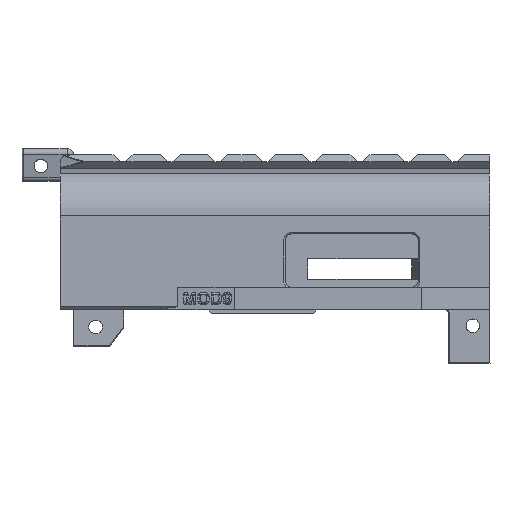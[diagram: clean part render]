
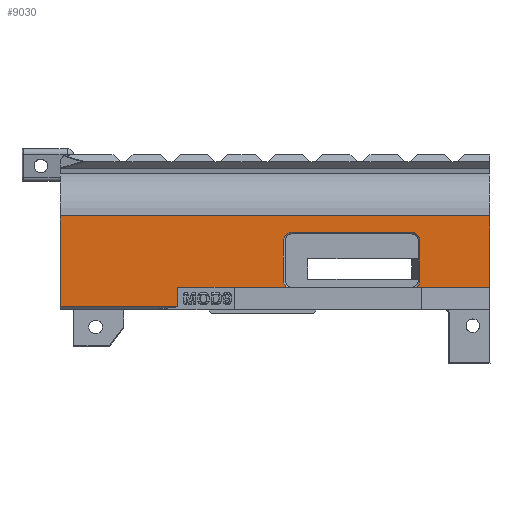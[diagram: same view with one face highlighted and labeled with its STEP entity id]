
A CAD part, top view. The second image highlights one B-rep face of the part: STEP entity #9030.
In plain terms, the highlighted planar face has unit normal (0, 0, 1).
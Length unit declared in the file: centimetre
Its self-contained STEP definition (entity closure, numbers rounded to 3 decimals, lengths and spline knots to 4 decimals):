
#732=LINE($,#12046,#1585);
#785=LINE($,#13323,#1638);
#786=LINE($,#13325,#1639);
#787=LINE($,#13328,#1640);
#788=LINE($,#13330,#1641);
#789=LINE($,#13332,#1642);
#790=LINE($,#13334,#1643);
#791=LINE($,#13336,#1644);
#792=LINE($,#13338,#1645);
#793=LINE($,#13342,#1646);
#794=LINE($,#13346,#1647);
#1585=VECTOR($,#10150,3.155);
#1638=VECTOR($,#10241,0.7183);
#1639=VECTOR($,#10242,1.0403);
#1640=VECTOR($,#10245,3.2523);
#1641=VECTOR($,#10246,19.0382);
#1642=VECTOR($,#10247,4.0257);
#1643=VECTOR($,#10248,5.189);
#1644=VECTOR($,#10249,0.8707);
#1645=VECTOR($,#10250,4.846);
#1646=VECTOR($,#10253,1.7606);
#1647=VECTOR($,#10256,5.2844);
#2394=PLANE($,#9542);
#2758=FACE_OUTER_BOUND($,#3283,.T.);
#3283=EDGE_LOOP($,(#6561,#6562,#6563,#6564,#6565,#6566,#6567,#6568,#6569,
#6570,#6571,#6572,#6573,#6574,#6575));
#3797=CIRCLE($,#9543,0.38);
#3798=CIRCLE($,#9544,0.38);
#3799=CIRCLE($,#9545,0.38);
#3800=CIRCLE($,#9546,0.38);
#3970=VERTEX_POINT($,#12043);
#3971=VERTEX_POINT($,#12045);
#4075=VERTEX_POINT($,#13321);
#4076=VERTEX_POINT($,#13322);
#4077=VERTEX_POINT($,#13324);
#4078=VERTEX_POINT($,#13326);
#4079=VERTEX_POINT($,#13329);
#4080=VERTEX_POINT($,#13331);
#4081=VERTEX_POINT($,#13333);
#4082=VERTEX_POINT($,#13335);
#4083=VERTEX_POINT($,#13337);
#4084=VERTEX_POINT($,#13339);
#4085=VERTEX_POINT($,#13341);
#4086=VERTEX_POINT($,#13343);
#4087=VERTEX_POINT($,#13345);
#4896=EDGE_CURVE($,#3971,#3970,#732,.T.);
#5046=EDGE_CURVE($,#4075,#4076,#785,.T.);
#5047=EDGE_CURVE($,#4077,#4075,#786,.T.);
#5048=EDGE_CURVE($,#4078,#4077,#3797,.T.);
#5049=EDGE_CURVE($,#3971,#4078,#787,.T.);
#5050=EDGE_CURVE($,#3970,#4079,#788,.T.);
#5051=EDGE_CURVE($,#4079,#4080,#789,.T.);
#5052=EDGE_CURVE($,#4081,#4080,#790,.T.);
#5053=EDGE_CURVE($,#4081,#4082,#791,.T.);
#5054=EDGE_CURVE($,#4083,#4082,#792,.T.);
#5055=EDGE_CURVE($,#4084,#4083,#3798,.T.);
#5056=EDGE_CURVE($,#4084,#4085,#793,.T.);
#5057=EDGE_CURVE($,#4086,#4085,#3799,.T.);
#5058=EDGE_CURVE($,#4087,#4086,#794,.T.);
#5059=EDGE_CURVE($,#4076,#4087,#3800,.T.);
#6561=ORIENTED_EDGE($,*,*,#5046,.F.);
#6562=ORIENTED_EDGE($,*,*,#5047,.F.);
#6563=ORIENTED_EDGE($,*,*,#5048,.F.);
#6564=ORIENTED_EDGE($,*,*,#5049,.F.);
#6565=ORIENTED_EDGE($,*,*,#4896,.T.);
#6566=ORIENTED_EDGE($,*,*,#5050,.T.);
#6567=ORIENTED_EDGE($,*,*,#5051,.T.);
#6568=ORIENTED_EDGE($,*,*,#5052,.F.);
#6569=ORIENTED_EDGE($,*,*,#5053,.T.);
#6570=ORIENTED_EDGE($,*,*,#5054,.F.);
#6571=ORIENTED_EDGE($,*,*,#5055,.F.);
#6572=ORIENTED_EDGE($,*,*,#5056,.T.);
#6573=ORIENTED_EDGE($,*,*,#5057,.F.);
#6574=ORIENTED_EDGE($,*,*,#5058,.F.);
#6575=ORIENTED_EDGE($,*,*,#5059,.F.);
#9030=ADVANCED_FACE($,(#2758),#2394,.T.);
#9542=AXIS2_PLACEMENT_3D($,#13320,#10239,#10240);
#9543=AXIS2_PLACEMENT_3D($,#13327,#10243,#10244);
#9544=AXIS2_PLACEMENT_3D($,#13340,#10251,#10252);
#9545=AXIS2_PLACEMENT_3D($,#13344,#10254,#10255);
#9546=AXIS2_PLACEMENT_3D($,#13347,#10257,#10258);
#10150=DIRECTION($,(0.,1.,0.));
#10239=DIRECTION('center_axis',(0.,0.,
1.));
#10240=DIRECTION('ref_axis',(0.,1.,0.));
#10241=DIRECTION($,(0.,1.,0.));
#10242=DIRECTION($,(0.,1.,0.));
#10243=DIRECTION('center_axis',(0.,0.,
1.));
#10244=DIRECTION('ref_axis',(0.707,-0.707,0.));
#10245=DIRECTION($,(-1.,0.,0.));
#10246=DIRECTION($,(-1.,0.,0.));
#10247=DIRECTION($,(0.,-1.,0.));
#10248=DIRECTION($,(-1.,0.,0.));
#10249=DIRECTION($,(0.,1.,0.));
#10250=DIRECTION($,(-1.,0.,0.));
#10251=DIRECTION('center_axis',(0.,0.,
1.));
#10252=DIRECTION('ref_axis',(-0.707,-0.707,0.));
#10253=DIRECTION($,(0.,1.,0.));
#10254=DIRECTION('center_axis',(0.,0.,
1.));
#10255=DIRECTION('ref_axis',(-0.707,0.707,0.));
#10256=DIRECTION($,(-1.,0.,0.));
#10257=DIRECTION('center_axis',(0.,0.,
1.));
#10258=DIRECTION('ref_axis',(0.707,0.707,0.));
#12043=CARTESIAN_POINT('',(1.1678,4.7361,2.11));
#12045=CARTESIAN_POINT('',(1.1678,1.5811,2.11));
#12046=CARTESIAN_POINT($,(1.1678,3.994,2.11));
#13320=CARTESIAN_POINT('Origin',(-0.3849,2.9869,2.11));
#13321=CARTESIAN_POINT('',(-1.9378,2.9214,2.11));
#13322=CARTESIAN_POINT('',(-1.9378,3.6397,2.11));
#13323=CARTESIAN_POINT($,(-1.9378,4.3379,2.11));
#13324=CARTESIAN_POINT('',(-1.9378,1.8811,2.11));
#13325=CARTESIAN_POINT($,(-1.9378,4.3379,2.11));
#13326=CARTESIAN_POINT('',(-2.0846,1.5811,2.11));
#13327=CARTESIAN_POINT('Origin',(-2.3178,1.8811,2.11));
#13328=CARTESIAN_POINT($,(-6.333,1.5811,2.11));
#13329=CARTESIAN_POINT('',(-17.8704,4.7361,2.11));
#13330=CARTESIAN_POINT($,(-2.0072,4.7361,2.11));
#13331=CARTESIAN_POINT('',(-17.8704,0.7104,2.11));
#13332=CARTESIAN_POINT($,(-17.8704,4.7361,2.11));
#13333=CARTESIAN_POINT('',(-12.6814,0.7104,2.11));
#13334=CARTESIAN_POINT($,(-5.4997,0.7104,2.11));
#13335=CARTESIAN_POINT('',(-12.6814,1.5811,2.11));
#13336=CARTESIAN_POINT($,(-12.6814,2.6586,2.11));
#13337=CARTESIAN_POINT('',(-7.8355,1.5811,2.11));
#13338=CARTESIAN_POINT($,(-6.333,1.5811,2.11));
#13339=CARTESIAN_POINT('',(-7.9822,1.8791,2.11));
#13340=CARTESIAN_POINT('Origin',(-7.6022,1.8811,2.11));
#13341=CARTESIAN_POINT('',(-7.9822,3.6397,2.11));
#13342=CARTESIAN_POINT($,(-7.9822,3.7226,2.11));
#13343=CARTESIAN_POINT('',(-7.6022,4.0197,2.11));
#13344=CARTESIAN_POINT('Origin',(-7.6022,3.6397,2.11));
#13345=CARTESIAN_POINT('',(-2.3178,4.0197,2.11));
#13346=CARTESIAN_POINT($,(-4.9547,4.0197,2.11));
#13347=CARTESIAN_POINT('Origin',(-2.3178,3.6397,2.11));
